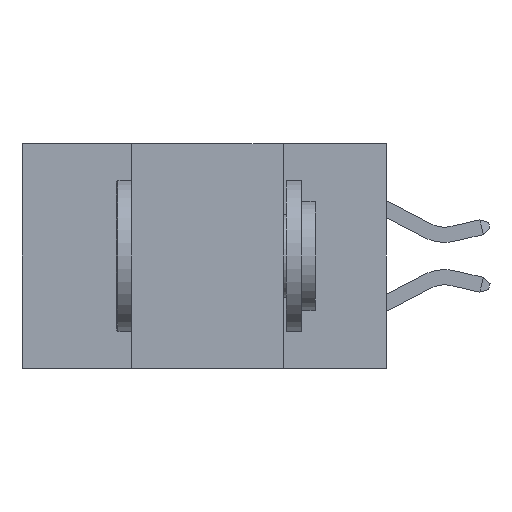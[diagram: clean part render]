
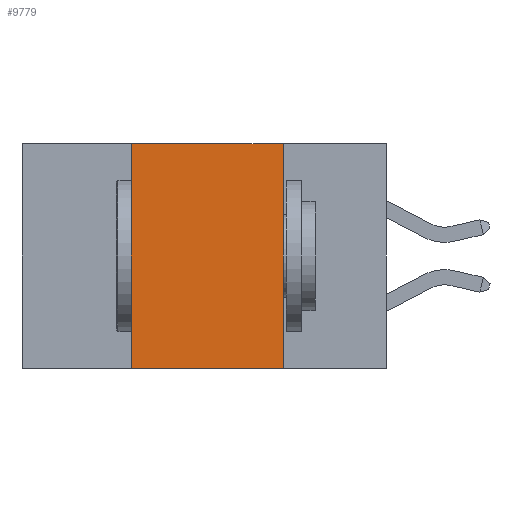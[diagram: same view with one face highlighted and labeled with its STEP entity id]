
A CAD part, left-side view. The second image highlights one B-rep face of the part: STEP entity #9779.
In plain terms, the highlighted planar face has unit normal (-1, 0, 0).
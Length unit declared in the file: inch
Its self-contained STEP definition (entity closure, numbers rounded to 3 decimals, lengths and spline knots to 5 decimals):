
#546 = CARTESIAN_POINT ( 'NONE',  ( 0., 0.17, 0. ) ) ;
#897 = DIRECTION ( 'NONE',  ( 0., 0., -1. ) ) ;
#943 = CARTESIAN_POINT ( 'NONE',  ( 0., 0.6, -0.37 ) ) ;
#1558 = DIRECTION ( 'NONE',  ( 0., -1., 0. ) ) ;
#2242 = ORIENTED_EDGE ( 'NONE', *, *, #7721, .F. ) ;
#2600 = DIRECTION ( 'NONE',  ( 0., 0., 1. ) ) ;
#2841 = PLANE ( 'NONE',  #11400 ) ;
#2914 = DIRECTION ( 'NONE',  ( 0., 0., -1. ) ) ;
#3176 = CARTESIAN_POINT ( 'NONE',  ( 0., 0.6, 0. ) ) ;
#4067 = LINE ( 'NONE', #943, #15153 ) ;
#4628 = DIRECTION ( 'NONE',  ( 0., -1., 0. ) ) ;
#4881 = ORIENTED_EDGE ( 'NONE', *, *, #18140, .T. ) ;
#5355 = FACE_OUTER_BOUND ( 'NONE', #15803, .T. ) ;
#5757 = CARTESIAN_POINT ( 'NONE',  ( 0., 0.6, 0. ) ) ;
#7721 = EDGE_CURVE ( 'NONE', #9893, #10792, #17451, .T. ) ;
#9779 = ADVANCED_FACE ( 'NONE', ( #5355 ), #2841, .F. ) ;
#9893 = VERTEX_POINT ( 'NONE', #14964 ) ;
#9976 = VECTOR ( 'NONE', #4628, 39.37008 ) ;
#10427 = VECTOR ( 'NONE', #897, 39.37008 ) ;
#10792 = VERTEX_POINT ( 'NONE', #546 ) ;
#11390 = VERTEX_POINT ( 'NONE', #15129 ) ;
#11400 = AXIS2_PLACEMENT_3D ( 'NONE', #5757, #17343, #2914 ) ;
#11451 = ORIENTED_EDGE ( 'NONE', *, *, #18451, .F. ) ;
#11509 = CARTESIAN_POINT ( 'NONE',  ( 0., 0.17, -0.37 ) ) ;
#13112 = VECTOR ( 'NONE', #2600, 39.37008 ) ;
#14083 = ORIENTED_EDGE ( 'NONE', *, *, #17853, .F. ) ;
#14347 = CARTESIAN_POINT ( 'NONE',  ( 0., 0.42, 0. ) ) ;
#14964 = CARTESIAN_POINT ( 'NONE',  ( 0., 0.42, 0. ) ) ;
#15129 = CARTESIAN_POINT ( 'NONE',  ( 0., 0.42, -0.37 ) ) ;
#15153 = VECTOR ( 'NONE', #1558, 39.37008 ) ;
#15803 = EDGE_LOOP ( 'NONE', ( #14083, #2242, #11451, #4881 ) ) ;
#16751 = LINE ( 'NONE', #16792, #10427 ) ;
#16792 = CARTESIAN_POINT ( 'NONE',  ( 0., 0.17, 0. ) ) ;
#16953 = LINE ( 'NONE', #14347, #13112 ) ;
#17343 = DIRECTION ( 'NONE',  ( 1., 0., 0. ) ) ;
#17379 = VERTEX_POINT ( 'NONE', #11509 ) ;
#17451 = LINE ( 'NONE', #3176, #9976 ) ;
#17853 = EDGE_CURVE ( 'NONE', #10792, #17379, #16751, .T. ) ;
#18140 = EDGE_CURVE ( 'NONE', #11390, #17379, #4067, .T. ) ;
#18451 = EDGE_CURVE ( 'NONE', #11390, #9893, #16953, .T. ) ;
